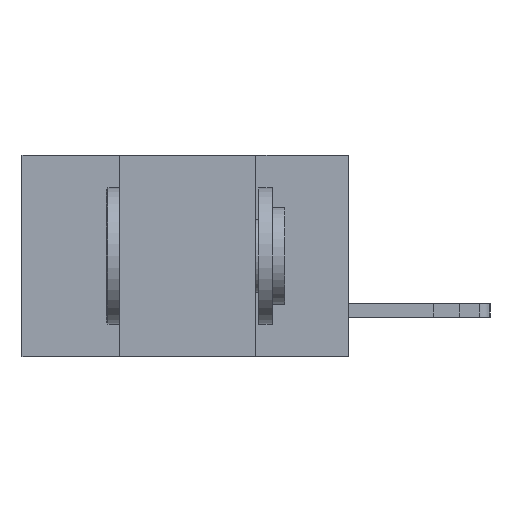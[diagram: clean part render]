
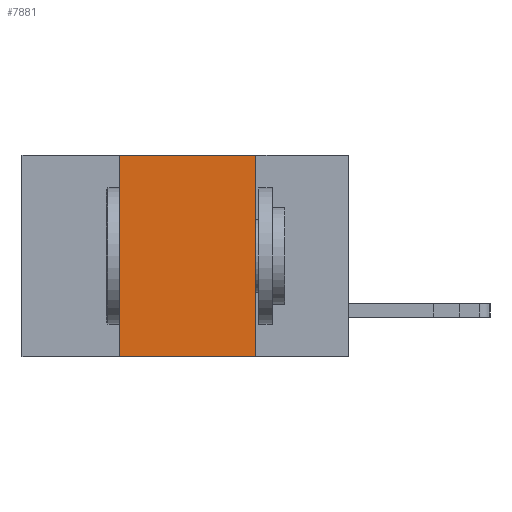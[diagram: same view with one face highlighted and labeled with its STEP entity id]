
A CAD part, left-side view. The second image highlights one B-rep face of the part: STEP entity #7881.
In plain terms, the highlighted planar face has unit normal (-1, 0, 0).
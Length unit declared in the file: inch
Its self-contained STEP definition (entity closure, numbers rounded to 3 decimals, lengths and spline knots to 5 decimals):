
#21 = VERTEX_POINT ( 'NONE', #5810 ) ;
#501 = EDGE_CURVE ( 'NONE', #19166, #12721, #13959, .T. ) ;
#927 = ORIENTED_EDGE ( 'NONE', *, *, #13621, .F. ) ;
#2559 = DIRECTION ( 'NONE',  ( 1., 0., 0. ) ) ;
#2578 = LINE ( 'NONE', #7319, #14669 ) ;
#2602 = VECTOR ( 'NONE', #17175, 39.37008 ) ;
#4456 = VERTEX_POINT ( 'NONE', #8241 ) ;
#5340 = LINE ( 'NONE', #6229, #2602 ) ;
#5810 = CARTESIAN_POINT ( 'NONE',  ( 0., 0.17, -0.37 ) ) ;
#6229 = CARTESIAN_POINT ( 'NONE',  ( 0., 0.6, 0. ) ) ;
#7099 = VECTOR ( 'NONE', #15518, 39.37008 ) ;
#7319 = CARTESIAN_POINT ( 'NONE',  ( 0., 0.6, -0.37 ) ) ;
#7331 = AXIS2_PLACEMENT_3D ( 'NONE', #11920, #2559, #13628 ) ;
#7881 = ADVANCED_FACE ( 'NONE', ( #15431 ), #12063, .F. ) ;
#8241 = CARTESIAN_POINT ( 'NONE',  ( 0., 0.17, 0. ) ) ;
#8422 = EDGE_LOOP ( 'NONE', ( #927, #13536, #17634, #14507 ) ) ;
#9408 = DIRECTION ( 'NONE',  ( 0., 0., 1. ) ) ;
#9908 = CARTESIAN_POINT ( 'NONE',  ( 0., 0.42, 0. ) ) ;
#10327 = LINE ( 'NONE', #20070, #7099 ) ;
#10509 = DIRECTION ( 'NONE',  ( 0., -1., 0. ) ) ;
#11920 = CARTESIAN_POINT ( 'NONE',  ( 0., 0.6, 0. ) ) ;
#12063 = PLANE ( 'NONE',  #7331 ) ;
#12721 = VERTEX_POINT ( 'NONE', #13333 ) ;
#13333 = CARTESIAN_POINT ( 'NONE',  ( 0., 0.42, 0. ) ) ;
#13536 = ORIENTED_EDGE ( 'NONE', *, *, #14301, .F. ) ;
#13621 = EDGE_CURVE ( 'NONE', #4456, #21, #10327, .T. ) ;
#13628 = DIRECTION ( 'NONE',  ( 0., 0., -1. ) ) ;
#13959 = LINE ( 'NONE', #9908, #14438 ) ;
#14276 = CARTESIAN_POINT ( 'NONE',  ( 0., 0.42, -0.37 ) ) ;
#14301 = EDGE_CURVE ( 'NONE', #12721, #4456, #5340, .T. ) ;
#14438 = VECTOR ( 'NONE', #9408, 39.37008 ) ;
#14507 = ORIENTED_EDGE ( 'NONE', *, *, #14646, .T. ) ;
#14646 = EDGE_CURVE ( 'NONE', #19166, #21, #2578, .T. ) ;
#14669 = VECTOR ( 'NONE', #10509, 39.37008 ) ;
#15431 = FACE_OUTER_BOUND ( 'NONE', #8422, .T. ) ;
#15518 = DIRECTION ( 'NONE',  ( 0., 0., -1. ) ) ;
#17175 = DIRECTION ( 'NONE',  ( 0., -1., 0. ) ) ;
#17634 = ORIENTED_EDGE ( 'NONE', *, *, #501, .F. ) ;
#19166 = VERTEX_POINT ( 'NONE', #14276 ) ;
#20070 = CARTESIAN_POINT ( 'NONE',  ( 0., 0.17, 0. ) ) ;
